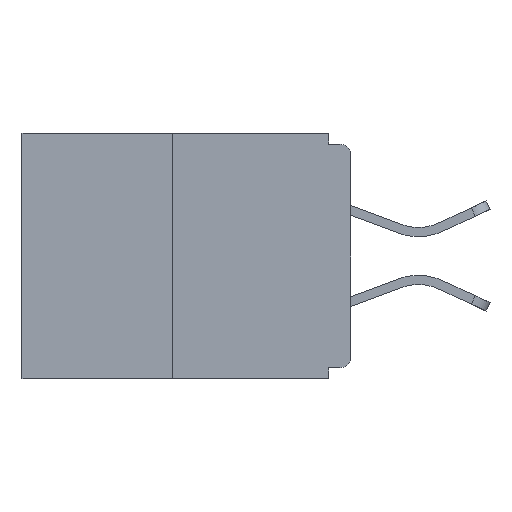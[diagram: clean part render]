
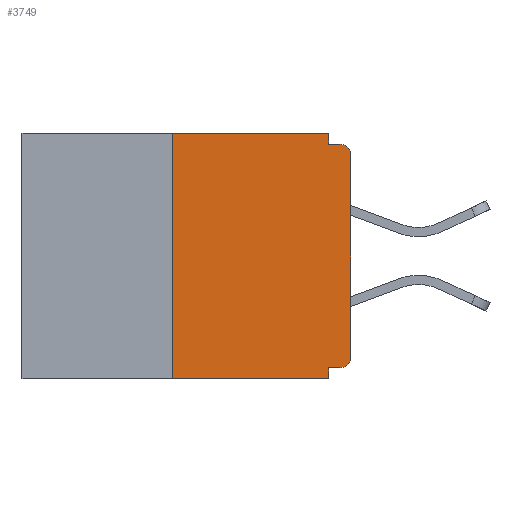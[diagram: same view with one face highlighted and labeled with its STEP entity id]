
A CAD part, left-side view. The second image highlights one B-rep face of the part: STEP entity #3749.
In plain terms, the highlighted planar face has unit normal (-1, 0, 0).
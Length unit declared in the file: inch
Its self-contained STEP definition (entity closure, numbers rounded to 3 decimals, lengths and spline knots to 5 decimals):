
#491 = CARTESIAN_POINT ( 'NONE',  ( 0., 0., -0.03 ) ) ;
#861 = VECTOR ( 'NONE', #7534, 39.37008 ) ;
#862 = VECTOR ( 'NONE', #5606, 39.37008 ) ;
#938 = VERTEX_POINT ( 'NONE', #5728 ) ;
#1103 = LINE ( 'NONE', #8037, #3645 ) ;
#1184 = DIRECTION ( 'NONE',  ( -1., 0., 0. ) ) ;
#1192 = VECTOR ( 'NONE', #5765, 39.37008 ) ;
#1246 = LINE ( 'NONE', #2645, #1401 ) ;
#1292 = EDGE_CURVE ( 'NONE', #3733, #13476, #9630, .T. ) ;
#1333 = DIRECTION ( 'NONE',  ( 0., 0., -1. ) ) ;
#1387 = ORIENTED_EDGE ( 'NONE', *, *, #1292, .F. ) ;
#1401 = VECTOR ( 'NONE', #7196, 39.37008 ) ;
#1409 = CARTESIAN_POINT ( 'NONE',  ( 0., 0., 0. ) ) ;
#1569 = DIRECTION ( 'NONE',  ( 0., 0., -1. ) ) ;
#1606 = EDGE_CURVE ( 'NONE', #4538, #8801, #2495, .T. ) ;
#1666 = ORIENTED_EDGE ( 'NONE', *, *, #8699, .F. ) ;
#1686 = CARTESIAN_POINT ( 'NONE',  ( 0., 0.46, -0.343 ) ) ;
#1722 = ORIENTED_EDGE ( 'NONE', *, *, #11057, .T. ) ;
#2495 = LINE ( 'NONE', #9087, #5761 ) ;
#2645 = CARTESIAN_POINT ( 'NONE',  ( 0., 0., -0.328 ) ) ;
#2885 = VERTEX_POINT ( 'NONE', #3931 ) ;
#3025 = EDGE_CURVE ( 'NONE', #8801, #3733, #1103, .T. ) ;
#3223 = CARTESIAN_POINT ( 'NONE',  ( 0., 0.015, -0.015 ) ) ;
#3258 = ORIENTED_EDGE ( 'NONE', *, *, #4802, .F. ) ;
#3644 = DIRECTION ( 'NONE',  ( 1., 0., 0. ) ) ;
#3645 = VECTOR ( 'NONE', #1333, 39.37008 ) ;
#3678 = EDGE_CURVE ( 'NONE', #8169, #7085, #5351, .T. ) ;
#3691 = DIRECTION ( 'NONE',  ( 0., 0., -1. ) ) ;
#3714 = CARTESIAN_POINT ( 'NONE',  ( 0., 0.015, -0.03 ) ) ;
#3733 = VERTEX_POINT ( 'NONE', #10217 ) ;
#3749 = ADVANCED_FACE ( 'NONE', ( #12055 ), #10395, .F. ) ;
#3931 = CARTESIAN_POINT ( 'NONE',  ( 0., 0.031, -0.328 ) ) ;
#4392 = EDGE_CURVE ( 'NONE', #938, #6844, #11861, .T. ) ;
#4538 = VERTEX_POINT ( 'NONE', #5271 ) ;
#4564 = DIRECTION ( 'NONE',  ( 0., 0., -1. ) ) ;
#4755 = AXIS2_PLACEMENT_3D ( 'NONE', #3714, #11443, #1569 ) ;
#4802 = EDGE_CURVE ( 'NONE', #2885, #6844, #12864, .T. ) ;
#5271 = CARTESIAN_POINT ( 'NONE',  ( 0., 0.25, 0. ) ) ;
#5351 = CIRCLE ( 'NONE', #11185, 0.015 ) ;
#5515 = VECTOR ( 'NONE', #10450, 39.37008 ) ;
#5606 = DIRECTION ( 'NONE',  ( 0., 0., -1. ) ) ;
#5686 = CARTESIAN_POINT ( 'NONE',  ( 0., 0.031, -0.343 ) ) ;
#5728 = CARTESIAN_POINT ( 'NONE',  ( 0., 0.25, -0.343 ) ) ;
#5761 = VECTOR ( 'NONE', #6922, 39.37008 ) ;
#5765 = DIRECTION ( 'NONE',  ( 0., 0., 1. ) ) ;
#6001 = VECTOR ( 'NONE', #9816, 39.37008 ) ;
#6341 = LINE ( 'NONE', #10598, #861 ) ;
#6531 = CARTESIAN_POINT ( 'NONE',  ( 0., 0., -0.015 ) ) ;
#6564 = AXIS2_PLACEMENT_3D ( 'NONE', #11460, #3644, #3691 ) ;
#6572 = CARTESIAN_POINT ( 'NONE',  ( 0., 0.015, -0.328 ) ) ;
#6579 = CARTESIAN_POINT ( 'NONE',  ( 0., 0.031, 0. ) ) ;
#6844 = VERTEX_POINT ( 'NONE', #5686 ) ;
#6922 = DIRECTION ( 'NONE',  ( 0., -1., 0. ) ) ;
#7085 = VERTEX_POINT ( 'NONE', #10965 ) ;
#7196 = DIRECTION ( 'NONE',  ( 0., 1., 0. ) ) ;
#7534 = DIRECTION ( 'NONE',  ( 0., 0., 1. ) ) ;
#8037 = CARTESIAN_POINT ( 'NONE',  ( 0., 0.031, 0. ) ) ;
#8169 = VERTEX_POINT ( 'NONE', #6572 ) ;
#8464 = ORIENTED_EDGE ( 'NONE', *, *, #3678, .T. ) ;
#8545 = CIRCLE ( 'NONE', #4755, 0.015 ) ;
#8699 = EDGE_CURVE ( 'NONE', #8169, #2885, #1246, .T. ) ;
#8801 = VERTEX_POINT ( 'NONE', #6579 ) ;
#8947 = ORIENTED_EDGE ( 'NONE', *, *, #10627, .F. ) ;
#9087 = CARTESIAN_POINT ( 'NONE',  ( 0., 0.46, 0. ) ) ;
#9331 = ORIENTED_EDGE ( 'NONE', *, *, #1606, .F. ) ;
#9630 = LINE ( 'NONE', #6531, #6001 ) ;
#9816 = DIRECTION ( 'NONE',  ( 0., -1., 0. ) ) ;
#10217 = CARTESIAN_POINT ( 'NONE',  ( 0., 0.031, -0.015 ) ) ;
#10395 = PLANE ( 'NONE',  #6564 ) ;
#10450 = DIRECTION ( 'NONE',  ( 0., -1., 0. ) ) ;
#10453 = VERTEX_POINT ( 'NONE', #491 ) ;
#10598 = CARTESIAN_POINT ( 'NONE',  ( 0., 0.25, 0. ) ) ;
#10627 = EDGE_CURVE ( 'NONE', #938, #4538, #6341, .T. ) ;
#10965 = CARTESIAN_POINT ( 'NONE',  ( 0., 0., -0.313 ) ) ;
#10967 = ORIENTED_EDGE ( 'NONE', *, *, #11323, .T. ) ;
#11057 = EDGE_CURVE ( 'NONE', #7085, #10453, #13215, .T. ) ;
#11185 = AXIS2_PLACEMENT_3D ( 'NONE', #12312, #1184, #4564 ) ;
#11323 = EDGE_CURVE ( 'NONE', #10453, #13476, #8545, .T. ) ;
#11443 = DIRECTION ( 'NONE',  ( -1., 0., 0. ) ) ;
#11460 = CARTESIAN_POINT ( 'NONE',  ( 0., 0.46, 0. ) ) ;
#11861 = LINE ( 'NONE', #1686, #5515 ) ;
#11994 = ORIENTED_EDGE ( 'NONE', *, *, #3025, .F. ) ;
#12055 = FACE_OUTER_BOUND ( 'NONE', #12389, .T. ) ;
#12312 = CARTESIAN_POINT ( 'NONE',  ( 0., 0.015, -0.313 ) ) ;
#12389 = EDGE_LOOP ( 'NONE', ( #9331, #8947, #12596, #3258, #1666, #8464, #1722, #10967, #1387, #11994 ) ) ;
#12596 = ORIENTED_EDGE ( 'NONE', *, *, #4392, .T. ) ;
#12864 = LINE ( 'NONE', #14158, #862 ) ;
#13215 = LINE ( 'NONE', #1409, #1192 ) ;
#13476 = VERTEX_POINT ( 'NONE', #3223 ) ;
#14158 = CARTESIAN_POINT ( 'NONE',  ( 0., 0.031, -0.343 ) ) ;
